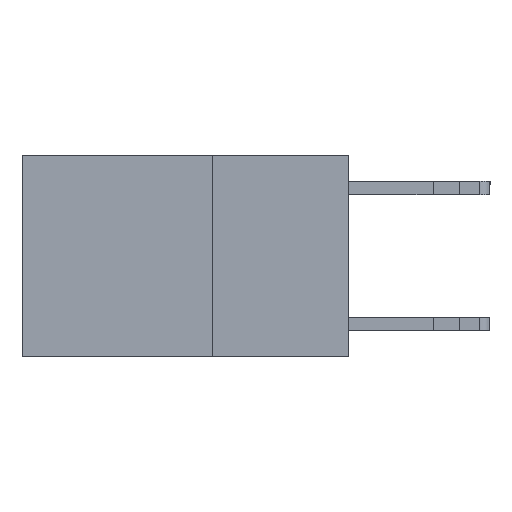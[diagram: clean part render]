
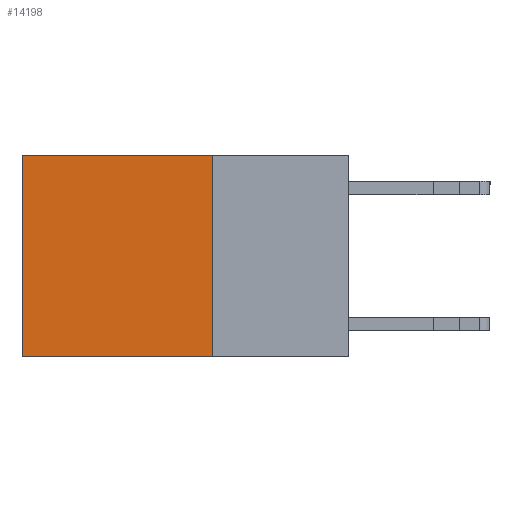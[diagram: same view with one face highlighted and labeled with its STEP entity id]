
A CAD part, left-side view. The second image highlights one B-rep face of the part: STEP entity #14198.
In plain terms, the highlighted planar face has unit normal (-1, 0, 0).
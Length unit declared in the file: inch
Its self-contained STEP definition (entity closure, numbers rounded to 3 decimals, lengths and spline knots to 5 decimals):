
#3475 = DIRECTION ( 'NONE',  ( 0., 0., -1. ) ) ;
#3922 = LINE ( 'NONE', #19797, #21679 ) ;
#4480 = LINE ( 'NONE', #15428, #18153 ) ;
#4503 = EDGE_LOOP ( 'NONE', ( #19266, #8508, #21216, #7718 ) ) ;
#5362 = VECTOR ( 'NONE', #17394, 39.37008 ) ;
#5752 = CARTESIAN_POINT ( 'NONE',  ( 0.2625, 0.25, 0. ) ) ;
#6863 = DIRECTION ( 'NONE',  ( 1., 0., 0. ) ) ;
#7718 = ORIENTED_EDGE ( 'NONE', *, *, #22647, .T. ) ;
#8508 = ORIENTED_EDGE ( 'NONE', *, *, #9893, .F. ) ;
#9018 = DIRECTION ( 'NONE',  ( 0., 1., 0. ) ) ;
#9893 = EDGE_CURVE ( 'NONE', #16814, #15741, #12284, .T. ) ;
#10418 = AXIS2_PLACEMENT_3D ( 'NONE', #12365, #6863, #3475 ) ;
#10424 = CARTESIAN_POINT ( 'NONE',  ( 0.2625, 0.25, -0.37 ) ) ;
#11126 = LINE ( 'NONE', #14307, #13262 ) ;
#12284 = LINE ( 'NONE', #15513, #5362 ) ;
#12365 = CARTESIAN_POINT ( 'NONE',  ( 0.2625, 0.25, 0. ) ) ;
#13262 = VECTOR ( 'NONE', #9018, 39.37008 ) ;
#14198 = ADVANCED_FACE ( 'NONE', ( #20685 ), #23198, .F. ) ;
#14307 = CARTESIAN_POINT ( 'NONE',  ( 0.2625, 0.25, 0. ) ) ;
#14409 = EDGE_CURVE ( 'NONE', #19212, #15741, #3922, .T. ) ;
#15428 = CARTESIAN_POINT ( 'NONE',  ( 0.2625, 0.25, 0. ) ) ;
#15513 = CARTESIAN_POINT ( 'NONE',  ( 0.2625, 0.25, -0.37 ) ) ;
#15741 = VERTEX_POINT ( 'NONE', #17106 ) ;
#16814 = VERTEX_POINT ( 'NONE', #10424 ) ;
#17106 = CARTESIAN_POINT ( 'NONE',  ( 0.2625, 0.6, -0.37 ) ) ;
#17394 = DIRECTION ( 'NONE',  ( 0., 1., 0. ) ) ;
#17904 = VERTEX_POINT ( 'NONE', #5752 ) ;
#18153 = VECTOR ( 'NONE', #22595, 39.37008 ) ;
#19212 = VERTEX_POINT ( 'NONE', #21645 ) ;
#19266 = ORIENTED_EDGE ( 'NONE', *, *, #14409, .T. ) ;
#19797 = CARTESIAN_POINT ( 'NONE',  ( 0.2625, 0.6, 0. ) ) ;
#20685 = FACE_OUTER_BOUND ( 'NONE', #4503, .T. ) ;
#21216 = ORIENTED_EDGE ( 'NONE', *, *, #21763, .F. ) ;
#21645 = CARTESIAN_POINT ( 'NONE',  ( 0.2625, 0.6, 0. ) ) ;
#21679 = VECTOR ( 'NONE', #22022, 39.37008 ) ;
#21763 = EDGE_CURVE ( 'NONE', #17904, #16814, #4480, .T. ) ;
#22022 = DIRECTION ( 'NONE',  ( 0., 0., -1. ) ) ;
#22595 = DIRECTION ( 'NONE',  ( 0., 0., -1. ) ) ;
#22647 = EDGE_CURVE ( 'NONE', #17904, #19212, #11126, .T. ) ;
#23198 = PLANE ( 'NONE',  #10418 ) ;
